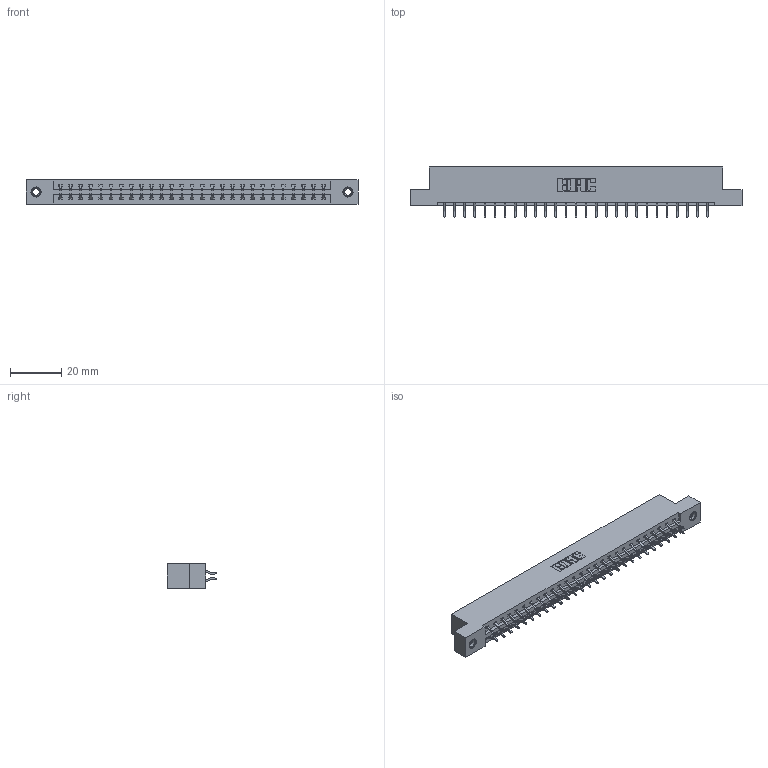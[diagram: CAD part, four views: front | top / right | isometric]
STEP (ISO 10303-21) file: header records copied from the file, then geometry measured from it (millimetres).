
FILE_DESCRIPTION (( 'STEP AP203' ), '1' );
FILE_NAME ('387-054-556-207.STEP', '2018-09-20T22:46:18', ( '' ), ( '' ), 'SwSTEP 2.0', 'SolidWorks 2016', '' );
FILE_SCHEMA (( 'CONFIG_CONTROL_DESIGN' ));
Length unit declared in the file: inch
Products named in the file (4): 337 Part_Flush Mounting Lugs - 0.156 Dia-TI; 345-292-001_556 Tail; 345-250-001_345-250-005-103; 387-054-556-207
Assembly tree (57 placements, depth 2):
  387-054-556-207
    337 Part_Flush Mounting Lugs - 0.156 Dia-TI
    345-292-001_556 Tail  x54
    345-250-001_345-250-005-103  x2
Bounding box: 130 x 19.57 x 9.4 mm (x, y, z)
Volume: 13484.8 mm3; surface area: 15077.9 mm2
Topology: 57 solids, 57 shells, 3414 faces, 10113 edges, 6662 vertices
Faces by surface type: plane 2370, cylinder 1028, cone 12, torus 4
Entity records: 24280 total; most frequent: CARTESIAN_POINT 4097, ORIENTED_EDGE 4014, DIRECTION 3533, EDGE_CURVE 2007, VECTOR 1851, LINE 1851, VERTEX_POINT 1332, AXIS2_PLACEMENT_3D 841
